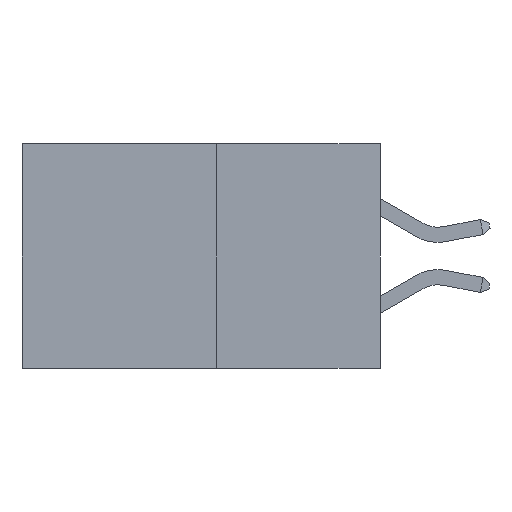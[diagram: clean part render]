
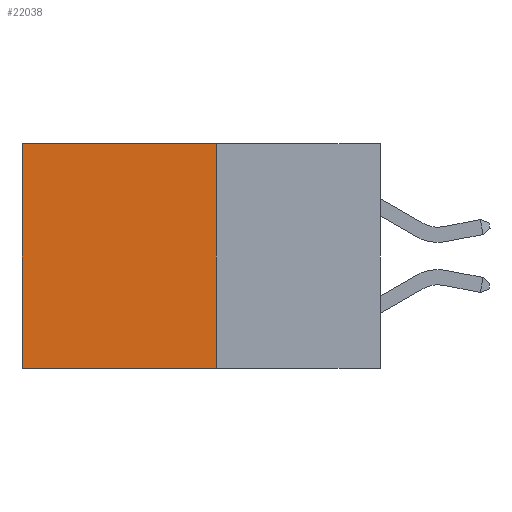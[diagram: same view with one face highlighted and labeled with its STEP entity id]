
A CAD part, left-side view. The second image highlights one B-rep face of the part: STEP entity #22038.
In plain terms, the highlighted planar face has unit normal (-1, 0, 0).
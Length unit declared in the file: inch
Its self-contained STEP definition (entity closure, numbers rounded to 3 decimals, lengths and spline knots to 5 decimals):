
#1367 = ORIENTED_EDGE ( 'NONE', *, *, #23893, .T. ) ;
#1798 = ORIENTED_EDGE ( 'NONE', *, *, #7753, .F. ) ;
#1880 = CARTESIAN_POINT ( 'NONE',  ( 0.277, 0.27, 0. ) ) ;
#3350 = VECTOR ( 'NONE', #24886, 39.37008 ) ;
#4109 = FACE_OUTER_BOUND ( 'NONE', #7509, .T. ) ;
#4292 = DIRECTION ( 'NONE',  ( 0., 1., 0. ) ) ;
#4724 = CARTESIAN_POINT ( 'NONE',  ( 0.277, 0.59, 0. ) ) ;
#4766 = ORIENTED_EDGE ( 'NONE', *, *, #8332, .F. ) ;
#4839 = LINE ( 'NONE', #29526, #3350 ) ;
#5915 = ORIENTED_EDGE ( 'NONE', *, *, #10937, .T. ) ;
#6407 = VECTOR ( 'NONE', #4292, 39.37008 ) ;
#7448 = VERTEX_POINT ( 'NONE', #4724 ) ;
#7509 = EDGE_LOOP ( 'NONE', ( #1367, #1798, #4766, #5915 ) ) ;
#7753 = EDGE_CURVE ( 'NONE', #14377, #13926, #4839, .T. ) ;
#8071 = PLANE ( 'NONE',  #10418 ) ;
#8332 = EDGE_CURVE ( 'NONE', #25895, #14377, #27240, .T. ) ;
#10418 = AXIS2_PLACEMENT_3D ( 'NONE', #24787, #10519, #27186 ) ;
#10519 = DIRECTION ( 'NONE',  ( 1., 0., 0. ) ) ;
#10937 = EDGE_CURVE ( 'NONE', #25895, #7448, #25505, .T. ) ;
#13079 = VECTOR ( 'NONE', #14657, 39.37008 ) ;
#13926 = VERTEX_POINT ( 'NONE', #26191 ) ;
#14377 = VERTEX_POINT ( 'NONE', #18584 ) ;
#14657 = DIRECTION ( 'NONE',  ( 0., 0., -1. ) ) ;
#17492 = DIRECTION ( 'NONE',  ( 0., 0., -1. ) ) ;
#18584 = CARTESIAN_POINT ( 'NONE',  ( 0.277, 0.27, -0.37 ) ) ;
#19985 = LINE ( 'NONE', #22390, #25548 ) ;
#21776 = CARTESIAN_POINT ( 'NONE',  ( 0.277, 0.27, -0.37 ) ) ;
#22038 = ADVANCED_FACE ( 'NONE', ( #4109 ), #8071, .F. ) ;
#22390 = CARTESIAN_POINT ( 'NONE',  ( 0.277, 0.59, -0.37 ) ) ;
#23893 = EDGE_CURVE ( 'NONE', #7448, #13926, #19985, .T. ) ;
#24787 = CARTESIAN_POINT ( 'NONE',  ( 0.277, 0.27, -0.37 ) ) ;
#24886 = DIRECTION ( 'NONE',  ( 0., 1., 0. ) ) ;
#25505 = LINE ( 'NONE', #1880, #6407 ) ;
#25548 = VECTOR ( 'NONE', #17492, 39.37008 ) ;
#25895 = VERTEX_POINT ( 'NONE', #28903 ) ;
#26191 = CARTESIAN_POINT ( 'NONE',  ( 0.277, 0.59, -0.37 ) ) ;
#27186 = DIRECTION ( 'NONE',  ( 0., 0., -1. ) ) ;
#27240 = LINE ( 'NONE', #21776, #13079 ) ;
#28903 = CARTESIAN_POINT ( 'NONE',  ( 0.277, 0.27, 0. ) ) ;
#29526 = CARTESIAN_POINT ( 'NONE',  ( 0.277, 0.27, -0.37 ) ) ;
